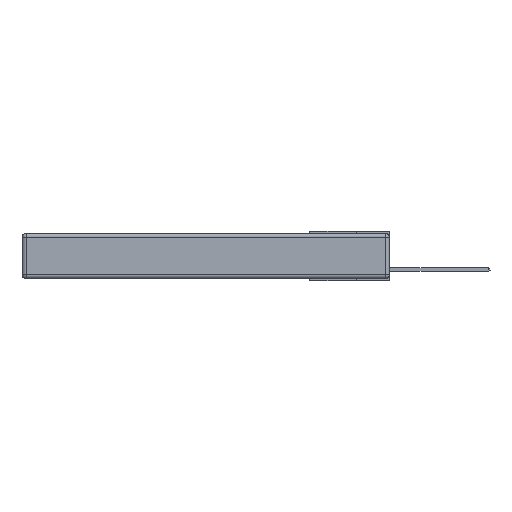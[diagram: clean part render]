
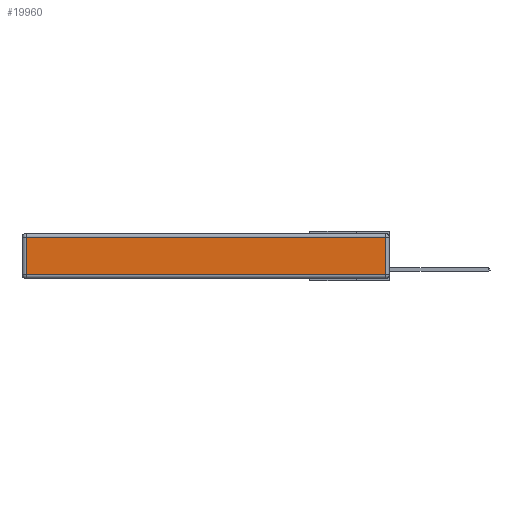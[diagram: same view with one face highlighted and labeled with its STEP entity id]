
A CAD part, left-side view. The second image highlights one B-rep face of the part: STEP entity #19960.
In plain terms, the highlighted planar face has unit normal (-1, 0, 0).
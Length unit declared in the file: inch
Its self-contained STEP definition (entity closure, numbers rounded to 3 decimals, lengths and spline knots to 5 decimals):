
#153 = DIRECTION ( 'NONE',  ( -1., 0., 0. ) ) ;
#535 = AXIS2_PLACEMENT_3D ( 'NONE', #18929, #153, #6905 ) ;
#722 = VECTOR ( 'NONE', #21518, 39.37008 ) ;
#760 = LINE ( 'NONE', #16721, #1836 ) ;
#1241 = LINE ( 'NONE', #5916, #722 ) ;
#1592 = VERTEX_POINT ( 'NONE', #13440 ) ;
#1662 = LINE ( 'NONE', #22306, #21678 ) ;
#1836 = VECTOR ( 'NONE', #7951, 39.37008 ) ;
#2290 = LINE ( 'NONE', #7410, #14958 ) ;
#2518 = EDGE_CURVE ( 'NONE', #1592, #10879, #1241, .T. ) ;
#2990 = ORIENTED_EDGE ( 'NONE', *, *, #4257, .T. ) ;
#3329 = DIRECTION ( 'NONE',  ( 0., 1., 0. ) ) ;
#3817 = EDGE_CURVE ( 'NONE', #10879, #17461, #760, .T. ) ;
#4257 = EDGE_CURVE ( 'NONE', #17461, #12477, #1662, .T. ) ;
#4428 = DIRECTION ( 'NONE',  ( 0., 0., -1. ) ) ;
#5607 = ORIENTED_EDGE ( 'NONE', *, *, #2518, .T. ) ;
#5916 = CARTESIAN_POINT ( 'NONE',  ( 0., 0., -0.313 ) ) ;
#6905 = DIRECTION ( 'NONE',  ( 0., 0., 1. ) ) ;
#7373 = CARTESIAN_POINT ( 'NONE',  ( 0., 0.03, -0.313 ) ) ;
#7410 = CARTESIAN_POINT ( 'NONE',  ( 0., 2.72, -0.343 ) ) ;
#7510 = ORIENTED_EDGE ( 'NONE', *, *, #8353, .T. ) ;
#7951 = DIRECTION ( 'NONE',  ( 0., 0., 1. ) ) ;
#8353 = EDGE_CURVE ( 'NONE', #12477, #1592, #2290, .T. ) ;
#8729 = EDGE_LOOP ( 'NONE', ( #5607, #21538, #2990, #7510 ) ) ;
#9798 = CARTESIAN_POINT ( 'NONE',  ( 0., 0.03, -0.03 ) ) ;
#10879 = VERTEX_POINT ( 'NONE', #7373 ) ;
#12110 = PLANE ( 'NONE',  #535 ) ;
#12477 = VERTEX_POINT ( 'NONE', #12931 ) ;
#12500 = FACE_OUTER_BOUND ( 'NONE', #8729, .T. ) ;
#12931 = CARTESIAN_POINT ( 'NONE',  ( 0., 2.72, -0.03 ) ) ;
#13440 = CARTESIAN_POINT ( 'NONE',  ( 0., 2.72, -0.313 ) ) ;
#14958 = VECTOR ( 'NONE', #4428, 39.37008 ) ;
#16721 = CARTESIAN_POINT ( 'NONE',  ( 0., 0.03, -0.343 ) ) ;
#17461 = VERTEX_POINT ( 'NONE', #9798 ) ;
#18929 = CARTESIAN_POINT ( 'NONE',  ( 0., 0., -0.343 ) ) ;
#19960 = ADVANCED_FACE ( 'NONE', ( #12500 ), #12110, .T. ) ;
#21518 = DIRECTION ( 'NONE',  ( 0., -1., 0. ) ) ;
#21538 = ORIENTED_EDGE ( 'NONE', *, *, #3817, .T. ) ;
#21678 = VECTOR ( 'NONE', #3329, 39.37008 ) ;
#22306 = CARTESIAN_POINT ( 'NONE',  ( 0., 2.75, -0.03 ) ) ;
